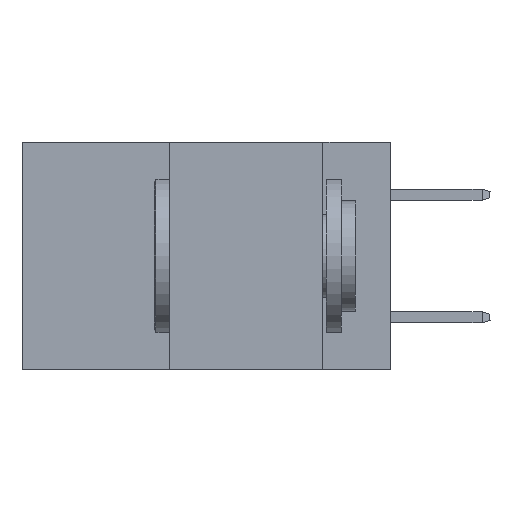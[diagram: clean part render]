
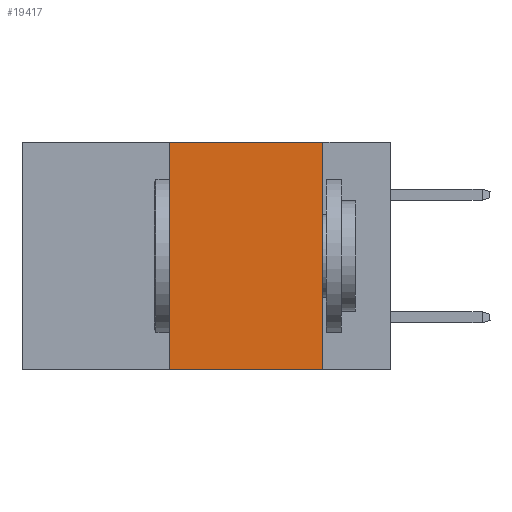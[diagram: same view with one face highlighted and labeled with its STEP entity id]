
A CAD part, left-side view. The second image highlights one B-rep face of the part: STEP entity #19417.
In plain terms, the highlighted planar face has unit normal (-1, 0, 0).
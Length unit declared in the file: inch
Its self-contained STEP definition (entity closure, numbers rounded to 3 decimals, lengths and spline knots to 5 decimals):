
#598 = CARTESIAN_POINT ( 'NONE',  ( 0., 0.6, 0. ) ) ;
#681 = DIRECTION ( 'NONE',  ( 0., 0., -1. ) ) ;
#1088 = CARTESIAN_POINT ( 'NONE',  ( 0., 0.36, 0. ) ) ;
#2187 = ORIENTED_EDGE ( 'NONE', *, *, #8743, .F. ) ;
#2393 = CARTESIAN_POINT ( 'NONE',  ( 0., 0.6, 0. ) ) ;
#2951 = CARTESIAN_POINT ( 'NONE',  ( 0., 0.11, 0. ) ) ;
#3754 = DIRECTION ( 'NONE',  ( 0., 0., -1. ) ) ;
#4005 = DIRECTION ( 'NONE',  ( 0., -1., 0. ) ) ;
#4466 = LINE ( 'NONE', #2393, #8549 ) ;
#6064 = EDGE_LOOP ( 'NONE', ( #12829, #9850, #2187, #21629 ) ) ;
#7730 = VERTEX_POINT ( 'NONE', #1088 ) ;
#7872 = DIRECTION ( 'NONE',  ( 1., 0., 0. ) ) ;
#8549 = VECTOR ( 'NONE', #4005, 39.37008 ) ;
#8743 = EDGE_CURVE ( 'NONE', #20498, #7730, #12018, .T. ) ;
#9416 = VERTEX_POINT ( 'NONE', #12141 ) ;
#9609 = CARTESIAN_POINT ( 'NONE',  ( 0., 0.6, -0.37 ) ) ;
#9720 = FACE_OUTER_BOUND ( 'NONE', #6064, .T. ) ;
#9850 = ORIENTED_EDGE ( 'NONE', *, *, #15275, .F. ) ;
#10736 = VERTEX_POINT ( 'NONE', #2951 ) ;
#12018 = LINE ( 'NONE', #18246, #17265 ) ;
#12141 = CARTESIAN_POINT ( 'NONE',  ( 0., 0.11, -0.37 ) ) ;
#12267 = EDGE_CURVE ( 'NONE', #20498, #9416, #19501, .T. ) ;
#12829 = ORIENTED_EDGE ( 'NONE', *, *, #18078, .F. ) ;
#14133 = AXIS2_PLACEMENT_3D ( 'NONE', #598, #7872, #681 ) ;
#15074 = CARTESIAN_POINT ( 'NONE',  ( 0., 0.11, 0. ) ) ;
#15275 = EDGE_CURVE ( 'NONE', #7730, #10736, #4466, .T. ) ;
#15303 = PLANE ( 'NONE',  #14133 ) ;
#16059 = DIRECTION ( 'NONE',  ( 0., 0., 1. ) ) ;
#17265 = VECTOR ( 'NONE', #16059, 39.37008 ) ;
#18078 = EDGE_CURVE ( 'NONE', #10736, #9416, #18538, .T. ) ;
#18246 = CARTESIAN_POINT ( 'NONE',  ( 0., 0.36, 0. ) ) ;
#18538 = LINE ( 'NONE', #15074, #19993 ) ;
#19417 = ADVANCED_FACE ( 'NONE', ( #9720 ), #15303, .F. ) ;
#19501 = LINE ( 'NONE', #9609, #20092 ) ;
#19993 = VECTOR ( 'NONE', #3754, 39.37008 ) ;
#20092 = VECTOR ( 'NONE', #23164, 39.37008 ) ;
#20498 = VERTEX_POINT ( 'NONE', #23204 ) ;
#21629 = ORIENTED_EDGE ( 'NONE', *, *, #12267, .T. ) ;
#23164 = DIRECTION ( 'NONE',  ( 0., -1., 0. ) ) ;
#23204 = CARTESIAN_POINT ( 'NONE',  ( 0., 0.36, -0.37 ) ) ;
